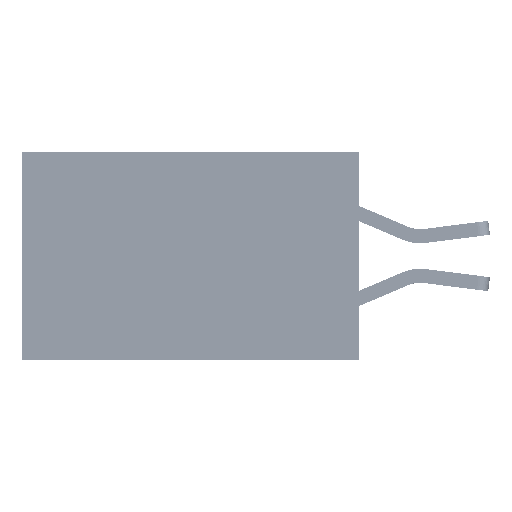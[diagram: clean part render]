
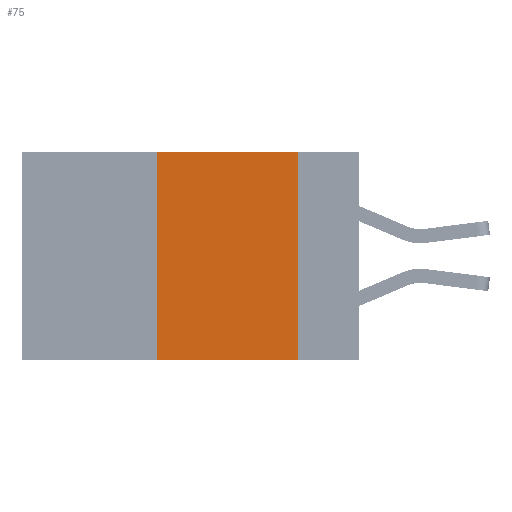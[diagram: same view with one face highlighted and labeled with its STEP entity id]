
A CAD part, left-side view. The second image highlights one B-rep face of the part: STEP entity #75.
In plain terms, the highlighted planar face has unit normal (-1, 0, 0).
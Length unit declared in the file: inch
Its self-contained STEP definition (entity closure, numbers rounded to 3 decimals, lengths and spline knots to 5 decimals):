
#75 = ADVANCED_FACE ( 'NONE', ( #23143 ), #17540, .F. ) ;
#3889 = AXIS2_PLACEMENT_3D ( 'NONE', #41998, #24126, #17990 ) ;
#5428 = ORIENTED_EDGE ( 'NONE', *, *, #27947, .T. ) ;
#11114 = EDGE_CURVE ( 'NONE', #32791, #30043, #38944, .T. ) ;
#11242 = CARTESIAN_POINT ( 'NONE',  ( 0., 0.6, -0.37 ) ) ;
#12041 = CARTESIAN_POINT ( 'NONE',  ( 0., 0.11, 0. ) ) ;
#17199 = VECTOR ( 'NONE', #18931, 39.37008 ) ;
#17540 = PLANE ( 'NONE',  #3889 ) ;
#17990 = DIRECTION ( 'NONE',  ( 0., 0., -1. ) ) ;
#18011 = VECTOR ( 'NONE', #31810, 39.37008 ) ;
#18603 = CARTESIAN_POINT ( 'NONE',  ( 0., 0.36, 0. ) ) ;
#18931 = DIRECTION ( 'NONE',  ( 0., -1., 0. ) ) ;
#19982 = CARTESIAN_POINT ( 'NONE',  ( 0., 0.11, 0. ) ) ;
#20294 = LINE ( 'NONE', #19982, #36059 ) ;
#22782 = ORIENTED_EDGE ( 'NONE', *, *, #46152, .F. ) ;
#22809 = DIRECTION ( 'NONE',  ( 0., 0., 1. ) ) ;
#23143 = FACE_OUTER_BOUND ( 'NONE', #42277, .T. ) ;
#24126 = DIRECTION ( 'NONE',  ( 1., 0., 0. ) ) ;
#24944 = EDGE_CURVE ( 'NONE', #30043, #25442, #27531, .T. ) ;
#25442 = VERTEX_POINT ( 'NONE', #12041 ) ;
#26717 = LINE ( 'NONE', #11242, #17199 ) ;
#27531 = LINE ( 'NONE', #45907, #18011 ) ;
#27947 = EDGE_CURVE ( 'NONE', #32791, #42396, #26717, .T. ) ;
#29395 = VECTOR ( 'NONE', #22809, 39.37008 ) ;
#30043 = VERTEX_POINT ( 'NONE', #41586 ) ;
#31810 = DIRECTION ( 'NONE',  ( 0., -1., 0. ) ) ;
#32253 = ORIENTED_EDGE ( 'NONE', *, *, #24944, .F. ) ;
#32791 = VERTEX_POINT ( 'NONE', #42245 ) ;
#34625 = CARTESIAN_POINT ( 'NONE',  ( 0., 0.11, -0.37 ) ) ;
#34972 = ORIENTED_EDGE ( 'NONE', *, *, #11114, .F. ) ;
#36059 = VECTOR ( 'NONE', #45082, 39.37008 ) ;
#38944 = LINE ( 'NONE', #18603, #29395 ) ;
#41586 = CARTESIAN_POINT ( 'NONE',  ( 0., 0.36, 0. ) ) ;
#41998 = CARTESIAN_POINT ( 'NONE',  ( 0., 0.6, 0. ) ) ;
#42245 = CARTESIAN_POINT ( 'NONE',  ( 0., 0.36, -0.37 ) ) ;
#42277 = EDGE_LOOP ( 'NONE', ( #22782, #32253, #34972, #5428 ) ) ;
#42396 = VERTEX_POINT ( 'NONE', #34625 ) ;
#45082 = DIRECTION ( 'NONE',  ( 0., 0., -1. ) ) ;
#45907 = CARTESIAN_POINT ( 'NONE',  ( 0., 0.6, 0. ) ) ;
#46152 = EDGE_CURVE ( 'NONE', #25442, #42396, #20294, .T. ) ;
